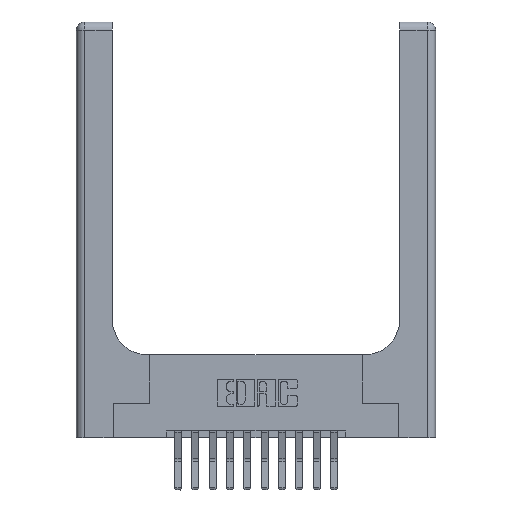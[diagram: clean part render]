
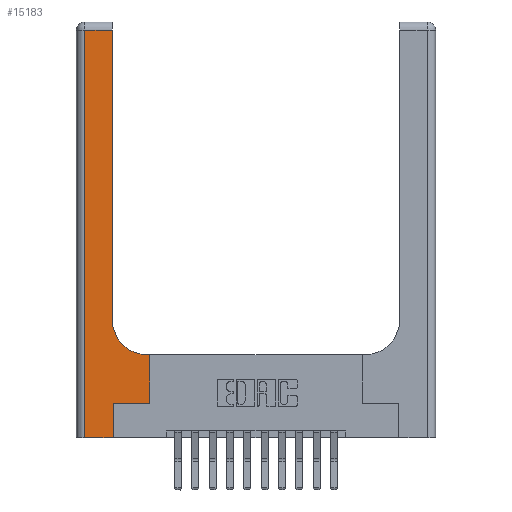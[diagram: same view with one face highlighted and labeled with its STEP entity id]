
A CAD part, top view. The second image highlights one B-rep face of the part: STEP entity #15183.
In plain terms, the highlighted planar face has unit normal (0, 0, 1).
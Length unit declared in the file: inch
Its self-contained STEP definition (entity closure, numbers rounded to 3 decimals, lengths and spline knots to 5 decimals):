
#187 = CARTESIAN_POINT ( 'NONE',  ( 0.528, 0.6, 0.37 ) ) ;
#762 = ORIENTED_EDGE ( 'NONE', *, *, #8077, .T. ) ;
#952 = VECTOR ( 'NONE', #9928, 39.37008 ) ;
#1759 = CARTESIAN_POINT ( 'NONE',  ( 0., 3., 0.37 ) ) ;
#2199 = CARTESIAN_POINT ( 'NONE',  ( 0.528, 0.25, 0.37 ) ) ;
#3006 = VERTEX_POINT ( 'NONE', #3457 ) ;
#3219 = LINE ( 'NONE', #13899, #15097 ) ;
#3457 = CARTESIAN_POINT ( 'NONE',  ( 0.265, 0.25, 0.37 ) ) ;
#3631 = VERTEX_POINT ( 'NONE', #13708 ) ;
#3733 = EDGE_LOOP ( 'NONE', ( #14530, #4030, #4251, #3790, #762, #11230, #6084, #7383, #9683 ) ) ;
#3790 = ORIENTED_EDGE ( 'NONE', *, *, #10392, .T. ) ;
#3846 = CARTESIAN_POINT ( 'NONE',  ( 0.26, 2.94, 0.37 ) ) ;
#4030 = ORIENTED_EDGE ( 'NONE', *, *, #5708, .T. ) ;
#4247 = LINE ( 'NONE', #2199, #14154 ) ;
#4251 = ORIENTED_EDGE ( 'NONE', *, *, #15566, .T. ) ;
#4333 = VERTEX_POINT ( 'NONE', #5470 ) ;
#4611 = DIRECTION ( 'NONE',  ( 0., 1., 0. ) ) ;
#4993 = EDGE_CURVE ( 'NONE', #15785, #4333, #12637, .T. ) ;
#5224 = CARTESIAN_POINT ( 'NONE',  ( 0., 0., 0.37 ) ) ;
#5371 = VERTEX_POINT ( 'NONE', #3846 ) ;
#5470 = CARTESIAN_POINT ( 'NONE',  ( 0.51, 0.6, 0.37 ) ) ;
#5576 = DIRECTION ( 'NONE',  ( 1., 0., 0. ) ) ;
#5617 = VERTEX_POINT ( 'NONE', #15792 ) ;
#5708 = EDGE_CURVE ( 'NONE', #5371, #8837, #7201, .T. ) ;
#6084 = ORIENTED_EDGE ( 'NONE', *, *, #6750, .T. ) ;
#6474 = DIRECTION ( 'NONE',  ( 1., 0., 0. ) ) ;
#6750 = EDGE_CURVE ( 'NONE', #13326, #15785, #4247, .T. ) ;
#6754 = DIRECTION ( 'NONE',  ( 1., 0., 0. ) ) ;
#7201 = LINE ( 'NONE', #7447, #9515 ) ;
#7202 = VERTEX_POINT ( 'NONE', #14817 ) ;
#7343 = DIRECTION ( 'NONE',  ( -1., 0., 0. ) ) ;
#7349 = EDGE_CURVE ( 'NONE', #3006, #13326, #3219, .T. ) ;
#7383 = ORIENTED_EDGE ( 'NONE', *, *, #4993, .T. ) ;
#7447 = CARTESIAN_POINT ( 'NONE',  ( 0., 2.94, 0.37 ) ) ;
#7468 = AXIS2_PLACEMENT_3D ( 'NONE', #1759, #7867, #15393 ) ;
#7641 = CARTESIAN_POINT ( 'NONE',  ( 0.528, 0.25, 0.37 ) ) ;
#7860 = CARTESIAN_POINT ( 'NONE',  ( 0.265, 0., 0.37 ) ) ;
#7867 = DIRECTION ( 'NONE',  ( 0., 0., -1. ) ) ;
#8077 = EDGE_CURVE ( 'NONE', #7202, #3006, #10009, .T. ) ;
#8763 = DIRECTION ( 'NONE',  ( 0., -1., 0. ) ) ;
#8837 = VERTEX_POINT ( 'NONE', #14079 ) ;
#8881 = DIRECTION ( 'NONE',  ( 0., 1., 0. ) ) ;
#9133 = EDGE_CURVE ( 'NONE', #5617, #5371, #12146, .T. ) ;
#9377 = FACE_OUTER_BOUND ( 'NONE', #3733, .T. ) ;
#9515 = VECTOR ( 'NONE', #7343, 39.37008 ) ;
#9611 = CARTESIAN_POINT ( 'NONE',  ( 0.26, 3., 0.37 ) ) ;
#9683 = ORIENTED_EDGE ( 'NONE', *, *, #13101, .T. ) ;
#9804 = VECTOR ( 'NONE', #10878, 39.37008 ) ;
#9928 = DIRECTION ( 'NONE',  ( -1., 0., 0. ) ) ;
#10009 = LINE ( 'NONE', #7860, #10803 ) ;
#10392 = EDGE_CURVE ( 'NONE', #3631, #7202, #12799, .T. ) ;
#10803 = VECTOR ( 'NONE', #8881, 39.37008 ) ;
#10878 = DIRECTION ( 'NONE',  ( 0., 1., 0. ) ) ;
#11230 = ORIENTED_EDGE ( 'NONE', *, *, #7349, .T. ) ;
#11478 = VECTOR ( 'NONE', #6474, 39.37008 ) ;
#11514 = PLANE ( 'NONE',  #7468 ) ;
#11741 = DIRECTION ( 'NONE',  ( 0., 0., -1. ) ) ;
#11888 = LINE ( 'NONE', #13655, #12275 ) ;
#12119 = AXIS2_PLACEMENT_3D ( 'NONE', #14176, #11741, #6754 ) ;
#12146 = LINE ( 'NONE', #9611, #9804 ) ;
#12275 = VECTOR ( 'NONE', #8763, 39.37008 ) ;
#12383 = CARTESIAN_POINT ( 'NONE',  ( 0.26, 0.6, 0.37 ) ) ;
#12637 = LINE ( 'NONE', #12383, #952 ) ;
#12799 = LINE ( 'NONE', #5224, #11478 ) ;
#13101 = EDGE_CURVE ( 'NONE', #4333, #5617, #15821, .T. ) ;
#13326 = VERTEX_POINT ( 'NONE', #7641 ) ;
#13655 = CARTESIAN_POINT ( 'NONE',  ( 0.06, 3., 0.37 ) ) ;
#13708 = CARTESIAN_POINT ( 'NONE',  ( 0.06, 0., 0.37 ) ) ;
#13899 = CARTESIAN_POINT ( 'NONE',  ( 0.265, 0.25, 0.37 ) ) ;
#14079 = CARTESIAN_POINT ( 'NONE',  ( 0.06, 2.94, 0.37 ) ) ;
#14154 = VECTOR ( 'NONE', #4611, 39.37008 ) ;
#14176 = CARTESIAN_POINT ( 'NONE',  ( 0.51, 0.85, 0.37 ) ) ;
#14530 = ORIENTED_EDGE ( 'NONE', *, *, #9133, .T. ) ;
#14817 = CARTESIAN_POINT ( 'NONE',  ( 0.265, 0., 0.37 ) ) ;
#15097 = VECTOR ( 'NONE', #5576, 39.37008 ) ;
#15183 = ADVANCED_FACE ( 'NONE', ( #9377 ), #11514, .F. ) ;
#15393 = DIRECTION ( 'NONE',  ( -1., 0., 0. ) ) ;
#15566 = EDGE_CURVE ( 'NONE', #8837, #3631, #11888, .T. ) ;
#15785 = VERTEX_POINT ( 'NONE', #187 ) ;
#15792 = CARTESIAN_POINT ( 'NONE',  ( 0.26, 0.85, 0.37 ) ) ;
#15821 = CIRCLE ( 'NONE', #12119, 0.25 ) ;
